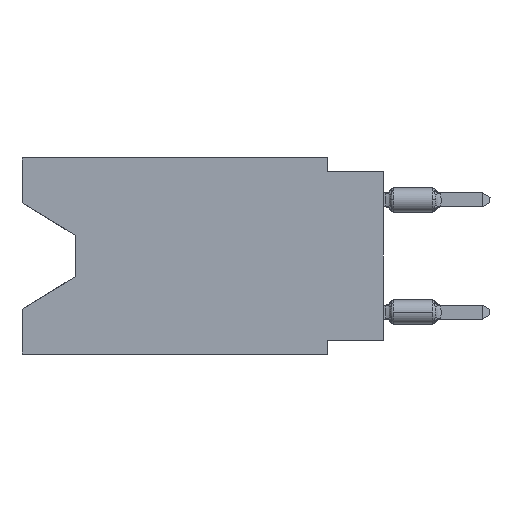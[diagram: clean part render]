
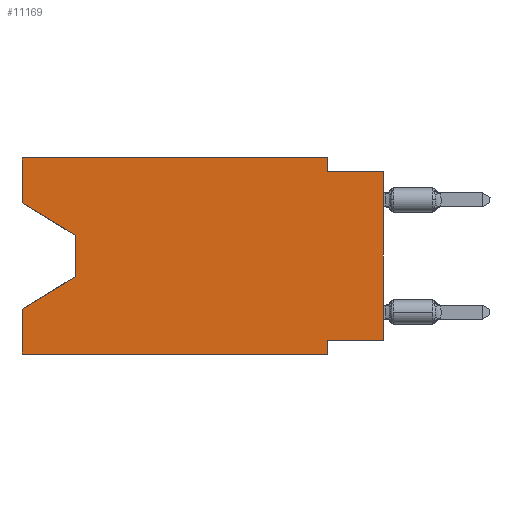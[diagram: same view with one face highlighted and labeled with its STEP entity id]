
A CAD part, left-side view. The second image highlights one B-rep face of the part: STEP entity #11169.
In plain terms, the highlighted planar face has unit normal (-1, 0, 0).
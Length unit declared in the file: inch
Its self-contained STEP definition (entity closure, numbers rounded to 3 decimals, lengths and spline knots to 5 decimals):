
#1360 = VERTEX_POINT ( 'NONE', #11541 ) ;
#1487 = EDGE_CURVE ( 'NONE', #25658, #9981, #18976, .T. ) ;
#1510 = CARTESIAN_POINT ( 'NONE',  ( 0., 0.645, 0. ) ) ;
#1663 = VECTOR ( 'NONE', #27327, 39.37008 ) ;
#1821 = CARTESIAN_POINT ( 'NONE',  ( 0., 0., -0.025 ) ) ;
#2035 = CARTESIAN_POINT ( 'NONE',  ( 0., 0.55, -0.212 ) ) ;
#2316 = DIRECTION ( 'NONE',  ( 0., 0.855, -0.519 ) ) ;
#3040 = CARTESIAN_POINT ( 'NONE',  ( 0., 0., -0.325 ) ) ;
#3268 = EDGE_CURVE ( 'NONE', #1360, #9973, #19330, .T. ) ;
#3659 = LINE ( 'NONE', #1510, #1663 ) ;
#3877 = LINE ( 'NONE', #12465, #16443 ) ;
#4214 = DIRECTION ( 'NONE',  ( 0., -0.855, -0.519 ) ) ;
#4255 = VECTOR ( 'NONE', #7782, 39.37008 ) ;
#4309 = LINE ( 'NONE', #17407, #25025 ) ;
#4658 = EDGE_LOOP ( 'NONE', ( #20934, #19053, #6157, #23964, #25196, #12237, #24494, #24490, #16201, #15513, #26960, #15644 ) ) ;
#5157 = EDGE_CURVE ( 'NONE', #21710, #1360, #3877, .T. ) ;
#5243 = EDGE_CURVE ( 'NONE', #5972, #10282, #19069, .T. ) ;
#5496 = VECTOR ( 'NONE', #6741, 39.37008 ) ;
#5972 = VERTEX_POINT ( 'NONE', #25629 ) ;
#6064 = CARTESIAN_POINT ( 'NONE',  ( 0., 0.55, -0.138 ) ) ;
#6085 = FACE_OUTER_BOUND ( 'NONE', #4658, .T. ) ;
#6149 = CARTESIAN_POINT ( 'NONE',  ( 0., 0., 0. ) ) ;
#6157 = ORIENTED_EDGE ( 'NONE', *, *, #14857, .T. ) ;
#6255 = DIRECTION ( 'NONE',  ( 0., 0., -1. ) ) ;
#6526 = VECTOR ( 'NONE', #6255, 39.37008 ) ;
#6741 = DIRECTION ( 'NONE',  ( 0., -1., 0. ) ) ;
#6775 = VECTOR ( 'NONE', #12628, 39.37008 ) ;
#6879 = CARTESIAN_POINT ( 'NONE',  ( 0., 0.645, -0.35 ) ) ;
#6975 = CARTESIAN_POINT ( 'NONE',  ( 0., 0.645, -0.26975 ) ) ;
#7318 = LINE ( 'NONE', #24931, #15592 ) ;
#7782 = DIRECTION ( 'NONE',  ( 0., -1., 0. ) ) ;
#8711 = LINE ( 'NONE', #23529, #13070 ) ;
#8753 = EDGE_CURVE ( 'NONE', #25658, #5972, #24465, .T. ) ;
#9870 = DIRECTION ( 'NONE',  ( 0., 0., -1. ) ) ;
#9973 = VERTEX_POINT ( 'NONE', #13979 ) ;
#9981 = VERTEX_POINT ( 'NONE', #1821 ) ;
#10085 = VERTEX_POINT ( 'NONE', #6064 ) ;
#10282 = VERTEX_POINT ( 'NONE', #12119 ) ;
#10289 = EDGE_CURVE ( 'NONE', #10085, #24199, #7318, .T. ) ;
#10744 = CARTESIAN_POINT ( 'NONE',  ( 0., 0.1, 0. ) ) ;
#11169 = ADVANCED_FACE ( 'NONE', ( #6085 ), #23426, .F. ) ;
#11541 = CARTESIAN_POINT ( 'NONE',  ( 0., 0.645, 0. ) ) ;
#11670 = CARTESIAN_POINT ( 'NONE',  ( 0., 0.1, -0.025 ) ) ;
#12119 = CARTESIAN_POINT ( 'NONE',  ( 0., 0.1, -0.35 ) ) ;
#12237 = ORIENTED_EDGE ( 'NONE', *, *, #5243, .F. ) ;
#12465 = CARTESIAN_POINT ( 'NONE',  ( 0., 0.645, 0. ) ) ;
#12628 = DIRECTION ( 'NONE',  ( 0., 0., 1. ) ) ;
#12697 = DIRECTION ( 'NONE',  ( 1., 0., 0. ) ) ;
#12720 = DIRECTION ( 'NONE',  ( 0., 0., 1. ) ) ;
#12967 = CARTESIAN_POINT ( 'NONE',  ( 0., 0.645, 0. ) ) ;
#13070 = VECTOR ( 'NONE', #4214, 39.37008 ) ;
#13979 = CARTESIAN_POINT ( 'NONE',  ( 0., 0.1, 0. ) ) ;
#13980 = EDGE_CURVE ( 'NONE', #20078, #9981, #18511, .T. ) ;
#14692 = CARTESIAN_POINT ( 'NONE',  ( 0., 0.645, 0. ) ) ;
#14695 = LINE ( 'NONE', #10744, #15283 ) ;
#14857 = EDGE_CURVE ( 'NONE', #24199, #17377, #4309, .T. ) ;
#15283 = VECTOR ( 'NONE', #23435, 39.37008 ) ;
#15513 = ORIENTED_EDGE ( 'NONE', *, *, #23331, .F. ) ;
#15592 = VECTOR ( 'NONE', #9870, 39.37008 ) ;
#15644 = ORIENTED_EDGE ( 'NONE', *, *, #5157, .F. ) ;
#16201 = ORIENTED_EDGE ( 'NONE', *, *, #13980, .F. ) ;
#16443 = VECTOR ( 'NONE', #12720, 39.37008 ) ;
#17131 = CARTESIAN_POINT ( 'NONE',  ( 0., 0.645, -0.08025 ) ) ;
#17281 = LINE ( 'NONE', #6879, #5496 ) ;
#17377 = VERTEX_POINT ( 'NONE', #6975 ) ;
#17407 = CARTESIAN_POINT ( 'NONE',  ( 0., 0.55, -0.212 ) ) ;
#17416 = AXIS2_PLACEMENT_3D ( 'NONE', #12967, #12697, #25266 ) ;
#17978 = EDGE_CURVE ( 'NONE', #27169, #17377, #3659, .T. ) ;
#18511 = LINE ( 'NONE', #27102, #4255 ) ;
#18625 = CARTESIAN_POINT ( 'NONE',  ( 0., 0., -0.325 ) ) ;
#18976 = LINE ( 'NONE', #6149, #6775 ) ;
#19053 = ORIENTED_EDGE ( 'NONE', *, *, #10289, .T. ) ;
#19069 = LINE ( 'NONE', #27660, #6526 ) ;
#19330 = LINE ( 'NONE', #14692, #19746 ) ;
#19746 = VECTOR ( 'NONE', #23018, 39.37008 ) ;
#20078 = VERTEX_POINT ( 'NONE', #11670 ) ;
#20825 = CARTESIAN_POINT ( 'NONE',  ( 0., 0.645, -0.35 ) ) ;
#20934 = ORIENTED_EDGE ( 'NONE', *, *, #24691, .T. ) ;
#21710 = VERTEX_POINT ( 'NONE', #17131 ) ;
#22353 = DIRECTION ( 'NONE',  ( 0., 1., 0. ) ) ;
#23018 = DIRECTION ( 'NONE',  ( 0., -1., 0. ) ) ;
#23331 = EDGE_CURVE ( 'NONE', #9973, #20078, #14695, .T. ) ;
#23426 = PLANE ( 'NONE',  #17416 ) ;
#23435 = DIRECTION ( 'NONE',  ( 0., 0., -1. ) ) ;
#23529 = CARTESIAN_POINT ( 'NONE',  ( 0., 0.645, -0.08025 ) ) ;
#23964 = ORIENTED_EDGE ( 'NONE', *, *, #17978, .F. ) ;
#24199 = VERTEX_POINT ( 'NONE', #2035 ) ;
#24465 = LINE ( 'NONE', #3040, #27662 ) ;
#24490 = ORIENTED_EDGE ( 'NONE', *, *, #1487, .T. ) ;
#24494 = ORIENTED_EDGE ( 'NONE', *, *, #8753, .F. ) ;
#24691 = EDGE_CURVE ( 'NONE', #21710, #10085, #8711, .T. ) ;
#24931 = CARTESIAN_POINT ( 'NONE',  ( 0., 0.55, -0.138 ) ) ;
#25025 = VECTOR ( 'NONE', #2316, 39.37008 ) ;
#25196 = ORIENTED_EDGE ( 'NONE', *, *, #26176, .T. ) ;
#25266 = DIRECTION ( 'NONE',  ( 0., 0., -1. ) ) ;
#25629 = CARTESIAN_POINT ( 'NONE',  ( 0., 0.1, -0.325 ) ) ;
#25658 = VERTEX_POINT ( 'NONE', #18625 ) ;
#26176 = EDGE_CURVE ( 'NONE', #27169, #10282, #17281, .T. ) ;
#26960 = ORIENTED_EDGE ( 'NONE', *, *, #3268, .F. ) ;
#27102 = CARTESIAN_POINT ( 'NONE',  ( 0., 0., -0.025 ) ) ;
#27169 = VERTEX_POINT ( 'NONE', #20825 ) ;
#27327 = DIRECTION ( 'NONE',  ( 0., 0., 1. ) ) ;
#27660 = CARTESIAN_POINT ( 'NONE',  ( 0., 0.1, -0.35 ) ) ;
#27662 = VECTOR ( 'NONE', #22353, 39.37008 ) ;
